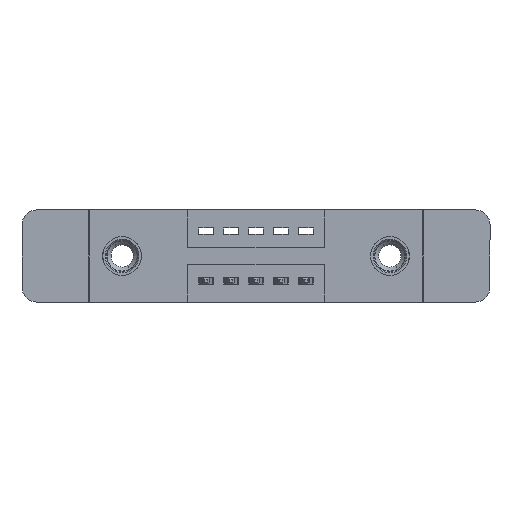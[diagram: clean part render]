
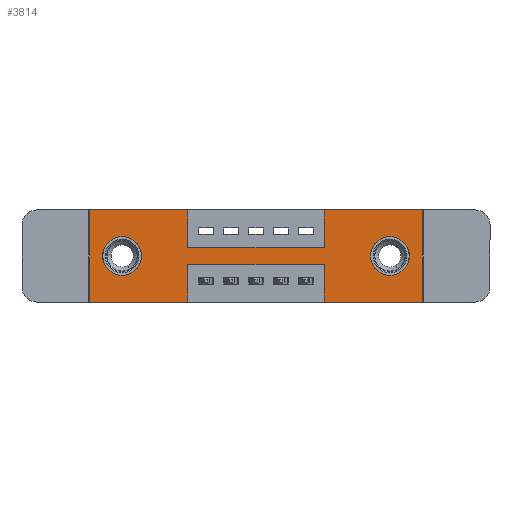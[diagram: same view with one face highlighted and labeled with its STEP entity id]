
A CAD part, front view. The second image highlights one B-rep face of the part: STEP entity #3814.
In plain terms, the highlighted planar face has unit normal (0, -1, 0).
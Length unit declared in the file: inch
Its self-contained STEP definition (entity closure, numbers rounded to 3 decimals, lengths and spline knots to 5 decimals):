
#42 = LINE ( 'NONE', #5015, #7284 ) ;
#63 = CARTESIAN_POINT ( 'NONE',  ( 0.3925, 0., -0.37 ) ) ;
#84 = VERTEX_POINT ( 'NONE', #13605 ) ;
#118 = CARTESIAN_POINT ( 'NONE',  ( 1.205, 0., -0.185 ) ) ;
#353 = CARTESIAN_POINT ( 'NONE',  ( 1.205, 0., -0.107 ) ) ;
#521 = CARTESIAN_POINT ( 'NONE',  ( 1.205, 0., -0.185 ) ) ;
#577 = EDGE_CURVE ( 'NONE', #3784, #895, #12467, .T. ) ;
#643 = CIRCLE ( 'NONE', #2579, 0.078 ) ;
#734 = DIRECTION ( 'NONE',  ( 0., 0., 1. ) ) ;
#773 = ORIENTED_EDGE ( 'NONE', *, *, #8982, .F. ) ;
#780 = CARTESIAN_POINT ( 'NONE',  ( 0.13, 0., -0.185 ) ) ;
#895 = VERTEX_POINT ( 'NONE', #10578 ) ;
#1105 = CARTESIAN_POINT ( 'NONE',  ( 0., 0., 0. ) ) ;
#1146 = CARTESIAN_POINT ( 'NONE',  ( 0.3925, 0., -0.37 ) ) ;
#1153 = ORIENTED_EDGE ( 'NONE', *, *, #2906, .F. ) ;
#1159 = VERTEX_POINT ( 'NONE', #7116 ) ;
#1439 = CARTESIAN_POINT ( 'NONE',  ( 0.3925, 0., -0.22 ) ) ;
#2040 = ORIENTED_EDGE ( 'NONE', *, *, #6744, .F. ) ;
#2072 = EDGE_CURVE ( 'NONE', #6891, #12402, #643, .T. ) ;
#2322 = CARTESIAN_POINT ( 'NONE',  ( 0., 0., -0.37 ) ) ;
#2390 = VERTEX_POINT ( 'NONE', #3287 ) ;
#2579 = AXIS2_PLACEMENT_3D ( 'NONE', #8790, #9883, #8844 ) ;
#2619 = FACE_OUTER_BOUND ( 'NONE', #10912, .T. ) ;
#2761 = EDGE_CURVE ( 'NONE', #1159, #12812, #13730, .T. ) ;
#2906 = EDGE_CURVE ( 'NONE', #5030, #11981, #3833, .T. ) ;
#3131 = EDGE_CURVE ( 'NONE', #6856, #4044, #10049, .T. ) ;
#3287 = CARTESIAN_POINT ( 'NONE',  ( 1.335, 0., 0. ) ) ;
#3348 = DIRECTION ( 'NONE',  ( 0., 0., -1. ) ) ;
#3409 = DIRECTION ( 'NONE',  ( -1., 0., 0. ) ) ;
#3675 = DIRECTION ( 'NONE',  ( -1., 0., 0. ) ) ;
#3737 = VECTOR ( 'NONE', #7302, 39.37008 ) ;
#3773 = CIRCLE ( 'NONE', #7126, 0.078 ) ;
#3784 = VERTEX_POINT ( 'NONE', #353 ) ;
#3814 = ADVANCED_FACE ( 'NONE', ( #5474, #7152, #2619 ), #9098, .T. ) ;
#3833 = LINE ( 'NONE', #1146, #8181 ) ;
#3883 = DIRECTION ( 'NONE',  ( 0., -1., 0. ) ) ;
#3954 = LINE ( 'NONE', #8576, #7129 ) ;
#3987 = ORIENTED_EDGE ( 'NONE', *, *, #3131, .F. ) ;
#4044 = VERTEX_POINT ( 'NONE', #9398 ) ;
#4110 = DIRECTION ( 'NONE',  ( 0., 0., -1. ) ) ;
#4307 = LINE ( 'NONE', #8863, #8851 ) ;
#4616 = CARTESIAN_POINT ( 'NONE',  ( 0.13, 0., -0.263 ) ) ;
#4617 = EDGE_LOOP ( 'NONE', ( #9910, #12661 ) ) ;
#4641 = EDGE_CURVE ( 'NONE', #84, #7401, #3954, .T. ) ;
#4730 = AXIS2_PLACEMENT_3D ( 'NONE', #521, #4820, #6071 ) ;
#4820 = DIRECTION ( 'NONE',  ( 0., 1., 0. ) ) ;
#4952 = CARTESIAN_POINT ( 'NONE',  ( 0.9425, 0., -0.37 ) ) ;
#4969 = ORIENTED_EDGE ( 'NONE', *, *, #7789, .F. ) ;
#5015 = CARTESIAN_POINT ( 'NONE',  ( 0.9425, 0., -0.37 ) ) ;
#5030 = VERTEX_POINT ( 'NONE', #1439 ) ;
#5111 = LINE ( 'NONE', #13289, #11520 ) ;
#5264 = CARTESIAN_POINT ( 'NONE',  ( 1.335, 0., 0. ) ) ;
#5265 = CARTESIAN_POINT ( 'NONE',  ( 0.3925, 0., 0. ) ) ;
#5474 = FACE_BOUND ( 'NONE', #4617, .T. ) ;
#5792 = VECTOR ( 'NONE', #13538, 39.37008 ) ;
#5826 = CARTESIAN_POINT ( 'NONE',  ( 0.3925, 0., -0.15 ) ) ;
#5887 = DIRECTION ( 'NONE',  ( 0., 0., -1. ) ) ;
#6026 = CARTESIAN_POINT ( 'NONE',  ( 0., 0., -0.37 ) ) ;
#6038 = ORIENTED_EDGE ( 'NONE', *, *, #2761, .F. ) ;
#6071 = DIRECTION ( 'NONE',  ( 0., 0., -1. ) ) ;
#6107 = LINE ( 'NONE', #5264, #10151 ) ;
#6119 = AXIS2_PLACEMENT_3D ( 'NONE', #118, #10911, #10959 ) ;
#6744 = EDGE_CURVE ( 'NONE', #11981, #6866, #9843, .T. ) ;
#6856 = VERTEX_POINT ( 'NONE', #8369 ) ;
#6866 = VERTEX_POINT ( 'NONE', #9185 ) ;
#6891 = VERTEX_POINT ( 'NONE', #4616 ) ;
#6940 = CARTESIAN_POINT ( 'NONE',  ( 0.9425, 0., 0. ) ) ;
#6962 = EDGE_CURVE ( 'NONE', #895, #3784, #10007, .T. ) ;
#7052 = ORIENTED_EDGE ( 'NONE', *, *, #7086, .F. ) ;
#7086 = EDGE_CURVE ( 'NONE', #11066, #5030, #5111, .T. ) ;
#7116 = CARTESIAN_POINT ( 'NONE',  ( 1.335, 0., -0.37 ) ) ;
#7126 = AXIS2_PLACEMENT_3D ( 'NONE', #780, #7261, #11147 ) ;
#7129 = VECTOR ( 'NONE', #11601, 39.37008 ) ;
#7141 = EDGE_LOOP ( 'NONE', ( #8045, #10756 ) ) ;
#7152 = FACE_BOUND ( 'NONE', #7141, .T. ) ;
#7258 = CARTESIAN_POINT ( 'NONE',  ( 0., 0., 0. ) ) ;
#7261 = DIRECTION ( 'NONE',  ( 0., 1., 0. ) ) ;
#7284 = VECTOR ( 'NONE', #734, 39.37008 ) ;
#7302 = DIRECTION ( 'NONE',  ( 1., 0., 0. ) ) ;
#7314 = EDGE_CURVE ( 'NONE', #12402, #6891, #3773, .T. ) ;
#7401 = VERTEX_POINT ( 'NONE', #6940 ) ;
#7789 = EDGE_CURVE ( 'NONE', #12812, #11066, #42, .T. ) ;
#8045 = ORIENTED_EDGE ( 'NONE', *, *, #7314, .T. ) ;
#8181 = VECTOR ( 'NONE', #3348, 39.37008 ) ;
#8348 = CARTESIAN_POINT ( 'NONE',  ( 0.13, 0., -0.107 ) ) ;
#8369 = CARTESIAN_POINT ( 'NONE',  ( 0., 0., 0. ) ) ;
#8430 = VERTEX_POINT ( 'NONE', #5826 ) ;
#8576 = CARTESIAN_POINT ( 'NONE',  ( 0.9425, 0., 0. ) ) ;
#8634 = DIRECTION ( 'NONE',  ( 1., 0., 0. ) ) ;
#8783 = VECTOR ( 'NONE', #4110, 39.37008 ) ;
#8790 = CARTESIAN_POINT ( 'NONE',  ( 0.13, 0., -0.185 ) ) ;
#8844 = DIRECTION ( 'NONE',  ( 0., 0., 1. ) ) ;
#8851 = VECTOR ( 'NONE', #11019, 39.37008 ) ;
#8863 = CARTESIAN_POINT ( 'NONE',  ( 0., 0., 0. ) ) ;
#8982 = EDGE_CURVE ( 'NONE', #4044, #8430, #9624, .T. ) ;
#8985 = ORIENTED_EDGE ( 'NONE', *, *, #4641, .F. ) ;
#8993 = ORIENTED_EDGE ( 'NONE', *, *, #9372, .F. ) ;
#9098 = PLANE ( 'NONE',  #11883 ) ;
#9185 = CARTESIAN_POINT ( 'NONE',  ( 0., 0., -0.37 ) ) ;
#9372 = EDGE_CURVE ( 'NONE', #8430, #84, #10133, .T. ) ;
#9395 = CARTESIAN_POINT ( 'NONE',  ( 0.3925, 0., -0.15 ) ) ;
#9398 = CARTESIAN_POINT ( 'NONE',  ( 0.3925, 0., 0. ) ) ;
#9624 = LINE ( 'NONE', #5265, #8783 ) ;
#9843 = LINE ( 'NONE', #6026, #5792 ) ;
#9883 = DIRECTION ( 'NONE',  ( 0., 1., 0. ) ) ;
#9910 = ORIENTED_EDGE ( 'NONE', *, *, #577, .T. ) ;
#10007 = CIRCLE ( 'NONE', #6119, 0.078 ) ;
#10049 = LINE ( 'NONE', #1105, #12235 ) ;
#10133 = LINE ( 'NONE', #9395, #3737 ) ;
#10151 = VECTOR ( 'NONE', #12787, 39.37008 ) ;
#10424 = VECTOR ( 'NONE', #12824, 39.37008 ) ;
#10578 = CARTESIAN_POINT ( 'NONE',  ( 1.205, 0., -0.263 ) ) ;
#10756 = ORIENTED_EDGE ( 'NONE', *, *, #2072, .T. ) ;
#10891 = VECTOR ( 'NONE', #3409, 39.37008 ) ;
#10911 = DIRECTION ( 'NONE',  ( 0., 1., 0. ) ) ;
#10912 = EDGE_LOOP ( 'NONE', ( #1153, #7052, #4969, #6038, #12335, #11422, #8985, #8993, #773, #3987, #13963, #2040 ) ) ;
#10925 = EDGE_CURVE ( 'NONE', #6866, #6856, #13945, .T. ) ;
#10959 = DIRECTION ( 'NONE',  ( 0., 0., -1. ) ) ;
#11019 = DIRECTION ( 'NONE',  ( 1., 0., 0. ) ) ;
#11066 = VERTEX_POINT ( 'NONE', #12104 ) ;
#11147 = DIRECTION ( 'NONE',  ( 0., 0., 1. ) ) ;
#11264 = CARTESIAN_POINT ( 'NONE',  ( 0., 0., -0.37 ) ) ;
#11422 = ORIENTED_EDGE ( 'NONE', *, *, #13159, .F. ) ;
#11520 = VECTOR ( 'NONE', #3675, 39.37008 ) ;
#11601 = DIRECTION ( 'NONE',  ( 0., 0., 1. ) ) ;
#11883 = AXIS2_PLACEMENT_3D ( 'NONE', #11264, #3883, #5887 ) ;
#11981 = VERTEX_POINT ( 'NONE', #63 ) ;
#12104 = CARTESIAN_POINT ( 'NONE',  ( 0.9425, 0., -0.22 ) ) ;
#12235 = VECTOR ( 'NONE', #8634, 39.37008 ) ;
#12335 = ORIENTED_EDGE ( 'NONE', *, *, #13569, .F. ) ;
#12402 = VERTEX_POINT ( 'NONE', #8348 ) ;
#12467 = CIRCLE ( 'NONE', #4730, 0.078 ) ;
#12661 = ORIENTED_EDGE ( 'NONE', *, *, #6962, .T. ) ;
#12787 = DIRECTION ( 'NONE',  ( 0., 0., -1. ) ) ;
#12812 = VERTEX_POINT ( 'NONE', #4952 ) ;
#12824 = DIRECTION ( 'NONE',  ( 0., 0., 1. ) ) ;
#13159 = EDGE_CURVE ( 'NONE', #7401, #2390, #4307, .T. ) ;
#13289 = CARTESIAN_POINT ( 'NONE',  ( 0.3925, 0., -0.22 ) ) ;
#13538 = DIRECTION ( 'NONE',  ( -1., 0., 0. ) ) ;
#13569 = EDGE_CURVE ( 'NONE', #2390, #1159, #6107, .T. ) ;
#13605 = CARTESIAN_POINT ( 'NONE',  ( 0.9425, 0., -0.15 ) ) ;
#13730 = LINE ( 'NONE', #2322, #10891 ) ;
#13945 = LINE ( 'NONE', #7258, #10424 ) ;
#13963 = ORIENTED_EDGE ( 'NONE', *, *, #10925, .F. ) ;
